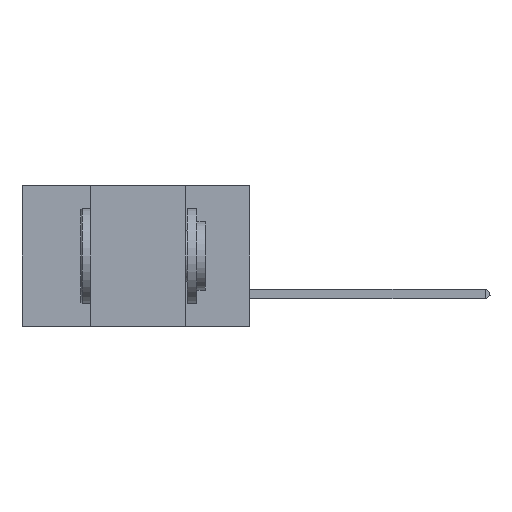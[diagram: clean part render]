
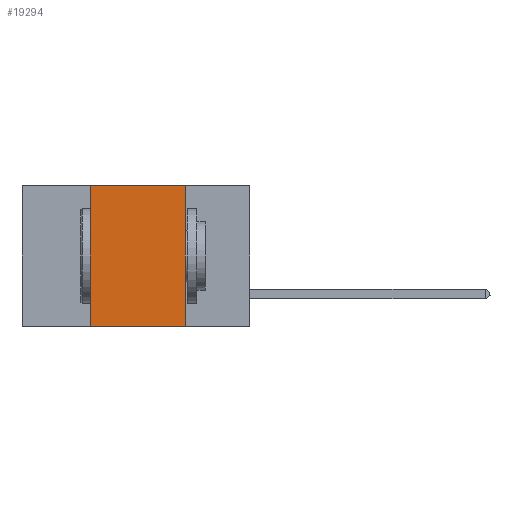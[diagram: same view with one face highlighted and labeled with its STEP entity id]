
A CAD part, left-side view. The second image highlights one B-rep face of the part: STEP entity #19294.
In plain terms, the highlighted planar face has unit normal (-1, 0, 0).
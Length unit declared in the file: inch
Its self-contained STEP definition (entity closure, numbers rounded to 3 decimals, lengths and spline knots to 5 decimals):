
#173 = VERTEX_POINT ( 'NONE', #21586 ) ;
#701 = EDGE_LOOP ( 'NONE', ( #1115, #48477, #31130, #38470 ) ) ;
#1115 = ORIENTED_EDGE ( 'NONE', *, *, #39103, .F. ) ;
#1891 = DIRECTION ( 'NONE',  ( 0., -1., 0. ) ) ;
#2892 = VECTOR ( 'NONE', #4323, 39.37008 ) ;
#4323 = DIRECTION ( 'NONE',  ( 0., -1., 0. ) ) ;
#6335 = CARTESIAN_POINT ( 'NONE',  ( 0., 0.6, 0. ) ) ;
#9823 = CARTESIAN_POINT ( 'NONE',  ( 0., 0.6, 0. ) ) ;
#9978 = DIRECTION ( 'NONE',  ( 1., 0., 0. ) ) ;
#13652 = VERTEX_POINT ( 'NONE', #47316 ) ;
#14384 = LINE ( 'NONE', #9823, #41649 ) ;
#15638 = AXIS2_PLACEMENT_3D ( 'NONE', #6335, #9978, #29097 ) ;
#15656 = EDGE_CURVE ( 'NONE', #23007, #173, #17784, .T. ) ;
#17784 = LINE ( 'NONE', #41856, #2892 ) ;
#17822 = PLANE ( 'NONE',  #15638 ) ;
#19294 = ADVANCED_FACE ( 'NONE', ( #32811 ), #17822, .F. ) ;
#21044 = DIRECTION ( 'NONE',  ( 0., 0., -1. ) ) ;
#21586 = CARTESIAN_POINT ( 'NONE',  ( 0., 0.17, -0.37 ) ) ;
#23007 = VERTEX_POINT ( 'NONE', #40287 ) ;
#23171 = VERTEX_POINT ( 'NONE', #30826 ) ;
#24376 = CARTESIAN_POINT ( 'NONE',  ( 0., 0.17, 0. ) ) ;
#29018 = LINE ( 'NONE', #24376, #42071 ) ;
#29097 = DIRECTION ( 'NONE',  ( 0., 0., -1. ) ) ;
#30575 = EDGE_CURVE ( 'NONE', #23007, #23171, #45246, .T. ) ;
#30826 = CARTESIAN_POINT ( 'NONE',  ( 0., 0.42, 0. ) ) ;
#31130 = ORIENTED_EDGE ( 'NONE', *, *, #30575, .F. ) ;
#32811 = FACE_OUTER_BOUND ( 'NONE', #701, .T. ) ;
#38470 = ORIENTED_EDGE ( 'NONE', *, *, #15656, .T. ) ;
#39103 = EDGE_CURVE ( 'NONE', #13652, #173, #29018, .T. ) ;
#40287 = CARTESIAN_POINT ( 'NONE',  ( 0., 0.42, -0.37 ) ) ;
#40418 = VECTOR ( 'NONE', #45881, 39.37008 ) ;
#41649 = VECTOR ( 'NONE', #1891, 39.37008 ) ;
#41856 = CARTESIAN_POINT ( 'NONE',  ( 0., 0.6, -0.37 ) ) ;
#42071 = VECTOR ( 'NONE', #21044, 39.37008 ) ;
#42847 = EDGE_CURVE ( 'NONE', #23171, #13652, #14384, .T. ) ;
#45246 = LINE ( 'NONE', #46212, #40418 ) ;
#45881 = DIRECTION ( 'NONE',  ( 0., 0., 1. ) ) ;
#46212 = CARTESIAN_POINT ( 'NONE',  ( 0., 0.42, 0. ) ) ;
#47316 = CARTESIAN_POINT ( 'NONE',  ( 0., 0.17, 0. ) ) ;
#48477 = ORIENTED_EDGE ( 'NONE', *, *, #42847, .F. ) ;
